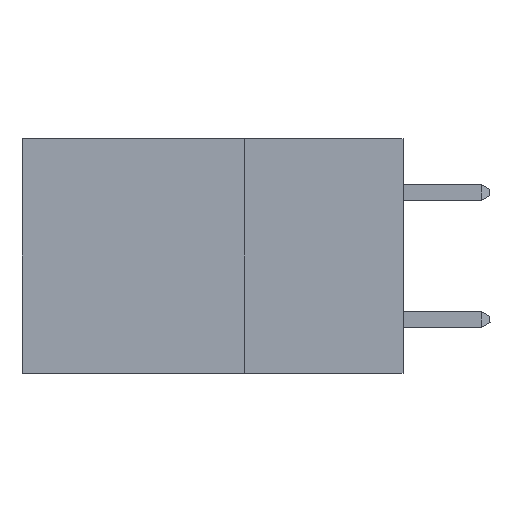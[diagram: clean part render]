
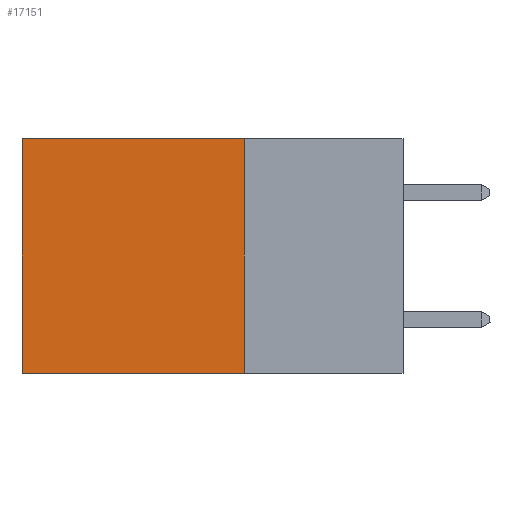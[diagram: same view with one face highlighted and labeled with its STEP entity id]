
A CAD part, left-side view. The second image highlights one B-rep face of the part: STEP entity #17151.
In plain terms, the highlighted planar face has unit normal (-1, 0, 0).
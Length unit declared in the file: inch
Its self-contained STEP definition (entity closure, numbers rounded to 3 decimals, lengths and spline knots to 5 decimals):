
#315 = VERTEX_POINT ( 'NONE', #16654 ) ;
#1987 = EDGE_CURVE ( 'NONE', #315, #15443, #32023, .T. ) ;
#2278 = LINE ( 'NONE', #16941, #10360 ) ;
#6256 = LINE ( 'NONE', #32278, #10315 ) ;
#7849 = CARTESIAN_POINT ( 'NONE',  ( 0.2875, 0.25, 0. ) ) ;
#8364 = CARTESIAN_POINT ( 'NONE',  ( 0.2875, 0.25, -0.37 ) ) ;
#8371 = DIRECTION ( 'NONE',  ( 0., 0., -1. ) ) ;
#8953 = DIRECTION ( 'NONE',  ( 0., 0., -1. ) ) ;
#10315 = VECTOR ( 'NONE', #12571, 39.37008 ) ;
#10360 = VECTOR ( 'NONE', #25597, 39.37008 ) ;
#11547 = ORIENTED_EDGE ( 'NONE', *, *, #29080, .F. ) ;
#12571 = DIRECTION ( 'NONE',  ( 0., 1., 0. ) ) ;
#14547 = DIRECTION ( 'NONE',  ( 1., 0., 0. ) ) ;
#15443 = VERTEX_POINT ( 'NONE', #28463 ) ;
#16654 = CARTESIAN_POINT ( 'NONE',  ( 0.2875, 0.6, 0. ) ) ;
#16941 = CARTESIAN_POINT ( 'NONE',  ( 0.2875, 0.25, 0. ) ) ;
#17151 = ADVANCED_FACE ( 'NONE', ( #20967 ), #28657, .F. ) ;
#19552 = CARTESIAN_POINT ( 'NONE',  ( 0.2875, 0.6, 0. ) ) ;
#19662 = ORIENTED_EDGE ( 'NONE', *, *, #30864, .F. ) ;
#20951 = VECTOR ( 'NONE', #8371, 39.37008 ) ;
#20967 = FACE_OUTER_BOUND ( 'NONE', #29731, .T. ) ;
#23597 = EDGE_CURVE ( 'NONE', #34082, #315, #2278, .T. ) ;
#24675 = ORIENTED_EDGE ( 'NONE', *, *, #1987, .T. ) ;
#25302 = VECTOR ( 'NONE', #36651, 39.37008 ) ;
#25597 = DIRECTION ( 'NONE',  ( 0., 1., 0. ) ) ;
#25687 = CARTESIAN_POINT ( 'NONE',  ( 0.2875, 0.25, 0. ) ) ;
#28463 = CARTESIAN_POINT ( 'NONE',  ( 0.2875, 0.6, -0.37 ) ) ;
#28657 = PLANE ( 'NONE',  #29224 ) ;
#29048 = CARTESIAN_POINT ( 'NONE',  ( 0.2875, 0.25, 0. ) ) ;
#29080 = EDGE_CURVE ( 'NONE', #30860, #15443, #6256, .T. ) ;
#29224 = AXIS2_PLACEMENT_3D ( 'NONE', #25687, #14547, #8953 ) ;
#29731 = EDGE_LOOP ( 'NONE', ( #24675, #11547, #19662, #30182 ) ) ;
#30182 = ORIENTED_EDGE ( 'NONE', *, *, #23597, .T. ) ;
#30860 = VERTEX_POINT ( 'NONE', #8364 ) ;
#30864 = EDGE_CURVE ( 'NONE', #34082, #30860, #33771, .T. ) ;
#32023 = LINE ( 'NONE', #19552, #20951 ) ;
#32278 = CARTESIAN_POINT ( 'NONE',  ( 0.2875, 0.25, -0.37 ) ) ;
#33771 = LINE ( 'NONE', #29048, #25302 ) ;
#34082 = VERTEX_POINT ( 'NONE', #7849 ) ;
#36651 = DIRECTION ( 'NONE',  ( 0., 0., -1. ) ) ;
